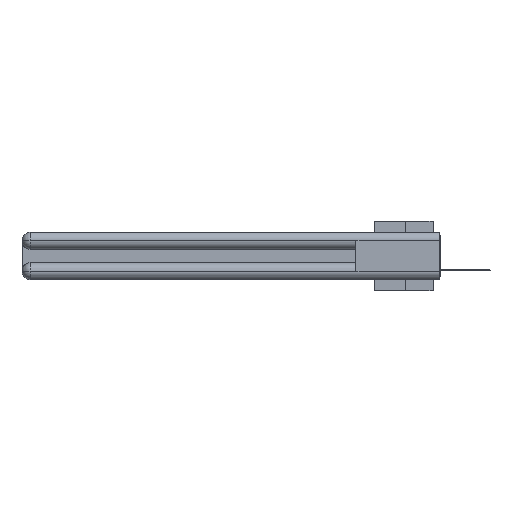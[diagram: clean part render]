
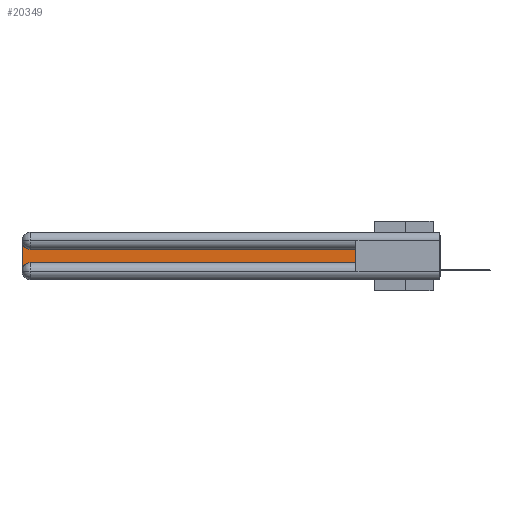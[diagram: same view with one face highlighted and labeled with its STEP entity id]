
A CAD part, left-side view. The second image highlights one B-rep face of the part: STEP entity #20349.
In plain terms, the highlighted planar face has unit normal (-1, 0, 0).
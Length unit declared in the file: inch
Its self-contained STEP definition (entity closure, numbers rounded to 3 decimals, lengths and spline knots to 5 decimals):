
#341 = EDGE_CURVE ( 'NONE', #18599, #3830, #16728, .T. ) ;
#2423 = PLANE ( 'NONE',  #12165 ) ;
#2430 = ORIENTED_EDGE ( 'NONE', *, *, #16016, .T. ) ;
#2585 = CARTESIAN_POINT ( 'NONE',  ( 0.075, 0.6, -0.2175 ) ) ;
#2743 = CARTESIAN_POINT ( 'NONE',  ( 0.075, 2.94, -0.0625 ) ) ;
#3830 = VERTEX_POINT ( 'NONE', #8338 ) ;
#3968 = LINE ( 'NONE', #2585, #10354 ) ;
#4120 = CARTESIAN_POINT ( 'NONE',  ( 0.075, 2.94, -0.1225 ) ) ;
#4289 = DIRECTION ( 'NONE',  ( 0., -1., 0. ) ) ;
#4667 = EDGE_CURVE ( 'NONE', #23524, #24046, #4748, .T. ) ;
#4748 = LINE ( 'NONE', #4764, #32549 ) ;
#4764 = CARTESIAN_POINT ( 'NONE',  ( 0.075, 0.6, -0.1225 ) ) ;
#5116 = EDGE_LOOP ( 'NONE', ( #7806, #7747, #13877, #2430, #11100, #25799 ) ) ;
#5276 = DIRECTION ( 'NONE',  ( 0., 0., -1. ) ) ;
#5317 = DIRECTION ( 'NONE',  ( 0., 0., 1. ) ) ;
#6416 = CIRCLE ( 'NONE', #14035, 0.06 ) ;
#7747 = ORIENTED_EDGE ( 'NONE', *, *, #16700, .T. ) ;
#7806 = ORIENTED_EDGE ( 'NONE', *, *, #4667, .T. ) ;
#8338 = CARTESIAN_POINT ( 'NONE',  ( 0.075, 0.6, -0.2175 ) ) ;
#8961 = VERTEX_POINT ( 'NONE', #12435 ) ;
#10354 = VECTOR ( 'NONE', #5317, 39.37008 ) ;
#11100 = ORIENTED_EDGE ( 'NONE', *, *, #341, .T. ) ;
#12083 = EDGE_CURVE ( 'NONE', #22811, #8961, #20990, .T. ) ;
#12165 = AXIS2_PLACEMENT_3D ( 'NONE', #18990, #21346, #29483 ) ;
#12435 = CARTESIAN_POINT ( 'NONE',  ( 0.075, 3., -0.2775 ) ) ;
#13877 = ORIENTED_EDGE ( 'NONE', *, *, #12083, .T. ) ;
#14035 = AXIS2_PLACEMENT_3D ( 'NONE', #2743, #24369, #16471 ) ;
#15695 = CARTESIAN_POINT ( 'NONE',  ( 0.075, 3., -0.0625 ) ) ;
#15894 = DIRECTION ( 'NONE',  ( 0., 0., -1. ) ) ;
#16016 = EDGE_CURVE ( 'NONE', #8961, #18599, #32641, .T. ) ;
#16329 = VECTOR ( 'NONE', #4289, 39.37008 ) ;
#16471 = DIRECTION ( 'NONE',  ( 0., 0., -1. ) ) ;
#16700 = EDGE_CURVE ( 'NONE', #24046, #22811, #6416, .T. ) ;
#16728 = LINE ( 'NONE', #20137, #16329 ) ;
#17361 = FACE_OUTER_BOUND ( 'NONE', #5116, .T. ) ;
#18599 = VERTEX_POINT ( 'NONE', #33845 ) ;
#18990 = CARTESIAN_POINT ( 'NONE',  ( 0.075, 3., -0.1225 ) ) ;
#20137 = CARTESIAN_POINT ( 'NONE',  ( 0.075, 0.6, -0.2175 ) ) ;
#20349 = ADVANCED_FACE ( 'NONE', ( #17361 ), #2423, .F. ) ;
#20990 = LINE ( 'NONE', #21141, #24339 ) ;
#21141 = CARTESIAN_POINT ( 'NONE',  ( 0.075, 3., -0.2175 ) ) ;
#21346 = DIRECTION ( 'NONE',  ( 1., 0., 0. ) ) ;
#22811 = VERTEX_POINT ( 'NONE', #15695 ) ;
#23524 = VERTEX_POINT ( 'NONE', #27344 ) ;
#24046 = VERTEX_POINT ( 'NONE', #4120 ) ;
#24339 = VECTOR ( 'NONE', #5276, 39.37008 ) ;
#24369 = DIRECTION ( 'NONE',  ( 1., 0., 0. ) ) ;
#25799 = ORIENTED_EDGE ( 'NONE', *, *, #32541, .T. ) ;
#27344 = CARTESIAN_POINT ( 'NONE',  ( 0.075, 0.6, -0.1225 ) ) ;
#29336 = DIRECTION ( 'NONE',  ( 1., 0., 0. ) ) ;
#29483 = DIRECTION ( 'NONE',  ( 0., 0., -1. ) ) ;
#29559 = CARTESIAN_POINT ( 'NONE',  ( 0.075, 2.94, -0.2775 ) ) ;
#32541 = EDGE_CURVE ( 'NONE', #3830, #23524, #3968, .T. ) ;
#32549 = VECTOR ( 'NONE', #33606, 39.37008 ) ;
#32601 = AXIS2_PLACEMENT_3D ( 'NONE', #29559, #29336, #15894 ) ;
#32641 = CIRCLE ( 'NONE', #32601, 0.06 ) ;
#33606 = DIRECTION ( 'NONE',  ( 0., 1., 0. ) ) ;
#33845 = CARTESIAN_POINT ( 'NONE',  ( 0.075, 2.94, -0.2175 ) ) ;
